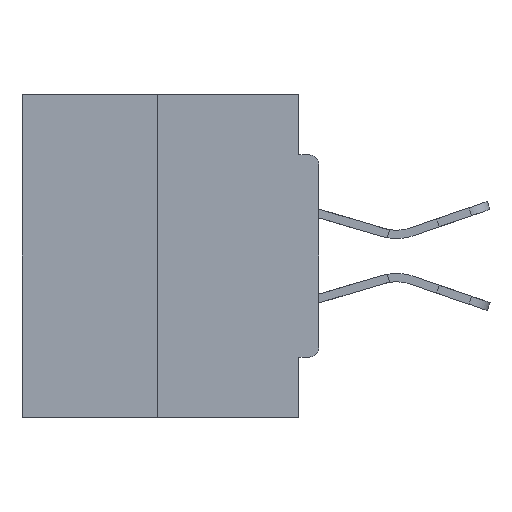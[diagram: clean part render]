
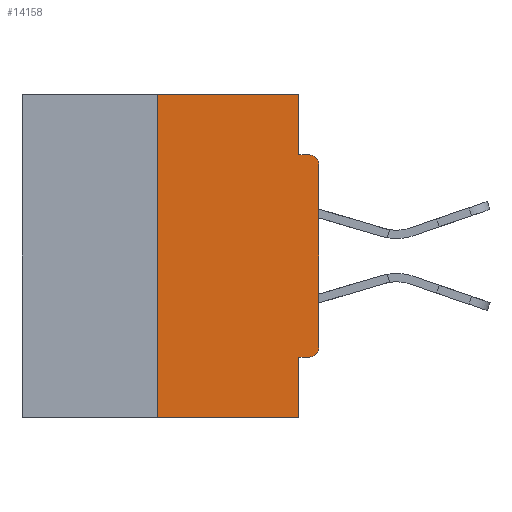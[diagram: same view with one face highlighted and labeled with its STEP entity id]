
A CAD part, left-side view. The second image highlights one B-rep face of the part: STEP entity #14158.
In plain terms, the highlighted planar face has unit normal (-1, 0, 0).
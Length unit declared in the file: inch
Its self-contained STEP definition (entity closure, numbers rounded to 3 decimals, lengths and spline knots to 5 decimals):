
#230 = ORIENTED_EDGE ( 'NONE', *, *, #789, .F. ) ;
#789 = EDGE_CURVE ( 'NONE', #2068, #12138, #25007, .T. ) ;
#1116 = VERTEX_POINT ( 'NONE', #14645 ) ;
#1739 = LINE ( 'NONE', #34316, #37080 ) ;
#1927 = CIRCLE ( 'NONE', #9295, 0.015 ) ;
#2068 = VERTEX_POINT ( 'NONE', #24907 ) ;
#2119 = DIRECTION ( 'NONE',  ( 0., 0., 1. ) ) ;
#2216 = EDGE_CURVE ( 'NONE', #1116, #17525, #6665, .T. ) ;
#2703 = EDGE_CURVE ( 'NONE', #25674, #12138, #1927, .T. ) ;
#2837 = CARTESIAN_POINT ( 'NONE',  ( 0., 0.25, 0. ) ) ;
#4883 = DIRECTION ( 'NONE',  ( -1., 0., 0. ) ) ;
#5009 = CARTESIAN_POINT ( 'NONE',  ( 0., 0., -0.4065 ) ) ;
#5109 = VECTOR ( 'NONE', #32019, 39.37008 ) ;
#5243 = ORIENTED_EDGE ( 'NONE', *, *, #34982, .T. ) ;
#5268 = DIRECTION ( 'NONE',  ( 0., 0., -1. ) ) ;
#5564 = ORIENTED_EDGE ( 'NONE', *, *, #30991, .F. ) ;
#6626 = ORIENTED_EDGE ( 'NONE', *, *, #29561, .T. ) ;
#6665 = LINE ( 'NONE', #30023, #23991 ) ;
#6961 = DIRECTION ( 'NONE',  ( 0., 0., -1. ) ) ;
#8534 = CARTESIAN_POINT ( 'NONE',  ( 0., 0.46, 0. ) ) ;
#9295 = AXIS2_PLACEMENT_3D ( 'NONE', #25380, #4883, #5268 ) ;
#9366 = DIRECTION ( 'NONE',  ( 0., 0., -1. ) ) ;
#9786 = EDGE_CURVE ( 'NONE', #11902, #2068, #20323, .T. ) ;
#11313 = ORIENTED_EDGE ( 'NONE', *, *, #35996, .T. ) ;
#11902 = VERTEX_POINT ( 'NONE', #14766 ) ;
#11984 = DIRECTION ( 'NONE',  ( 0., 0., -1. ) ) ;
#12138 = VERTEX_POINT ( 'NONE', #21803 ) ;
#12394 = CARTESIAN_POINT ( 'NONE',  ( 0., 0.031, -0.4065 ) ) ;
#12694 = ORIENTED_EDGE ( 'NONE', *, *, #2216, .F. ) ;
#12899 = PLANE ( 'NONE',  #28909 ) ;
#13634 = LINE ( 'NONE', #5009, #13907 ) ;
#13907 = VECTOR ( 'NONE', #25701, 39.37008 ) ;
#14158 = ADVANCED_FACE ( 'NONE', ( #21903 ), #12899, .F. ) ;
#14486 = DIRECTION ( 'NONE',  ( -1., 0., 0. ) ) ;
#14645 = CARTESIAN_POINT ( 'NONE',  ( 0., 0.25, -0.5 ) ) ;
#14766 = CARTESIAN_POINT ( 'NONE',  ( 0., 0.031, 0. ) ) ;
#15404 = CARTESIAN_POINT ( 'NONE',  ( 0., 0.46, 0. ) ) ;
#15468 = DIRECTION ( 'NONE',  ( 0., 0., 1. ) ) ;
#15965 = DIRECTION ( 'NONE',  ( 1., 0., 0. ) ) ;
#16001 = CARTESIAN_POINT ( 'NONE',  ( 0., 0., -0.0935 ) ) ;
#16078 = VECTOR ( 'NONE', #9366, 39.37008 ) ;
#16320 = VECTOR ( 'NONE', #20216, 39.37008 ) ;
#17525 = VERTEX_POINT ( 'NONE', #2837 ) ;
#17814 = LINE ( 'NONE', #29307, #16078 ) ;
#18212 = EDGE_CURVE ( 'NONE', #17525, #11902, #22536, .T. ) ;
#19085 = LINE ( 'NONE', #30772, #30173 ) ;
#20216 = DIRECTION ( 'NONE',  ( 0., -1., 0. ) ) ;
#20323 = LINE ( 'NONE', #26452, #5109 ) ;
#21071 = ORIENTED_EDGE ( 'NONE', *, *, #2703, .T. ) ;
#21586 = VERTEX_POINT ( 'NONE', #29163 ) ;
#21641 = CIRCLE ( 'NONE', #33888, 0.015 ) ;
#21744 = ORIENTED_EDGE ( 'NONE', *, *, #9786, .F. ) ;
#21803 = CARTESIAN_POINT ( 'NONE',  ( 0., 0.015, -0.0935 ) ) ;
#21903 = FACE_OUTER_BOUND ( 'NONE', #28185, .T. ) ;
#22145 = DIRECTION ( 'NONE',  ( 0., -1., 0. ) ) ;
#22536 = LINE ( 'NONE', #8534, #16320 ) ;
#23528 = VERTEX_POINT ( 'NONE', #29455 ) ;
#23991 = VECTOR ( 'NONE', #15468, 39.37008 ) ;
#24358 = ORIENTED_EDGE ( 'NONE', *, *, #34144, .F. ) ;
#24907 = CARTESIAN_POINT ( 'NONE',  ( 0., 0.031, -0.0935 ) ) ;
#25007 = LINE ( 'NONE', #16001, #30652 ) ;
#25380 = CARTESIAN_POINT ( 'NONE',  ( 0., 0.015, -0.1085 ) ) ;
#25674 = VERTEX_POINT ( 'NONE', #26966 ) ;
#25701 = DIRECTION ( 'NONE',  ( 0., 1., 0. ) ) ;
#26452 = CARTESIAN_POINT ( 'NONE',  ( 0., 0.031, 0. ) ) ;
#26966 = CARTESIAN_POINT ( 'NONE',  ( 0., 0., -0.1085 ) ) ;
#28185 = EDGE_LOOP ( 'NONE', ( #31526, #12694, #11313, #24358, #5564, #5243, #6626, #21071, #230, #21744 ) ) ;
#28909 = AXIS2_PLACEMENT_3D ( 'NONE', #15404, #15965, #6961 ) ;
#29163 = CARTESIAN_POINT ( 'NONE',  ( 0., 0.031, -0.5 ) ) ;
#29307 = CARTESIAN_POINT ( 'NONE',  ( 0., 0.031, -0.5 ) ) ;
#29455 = CARTESIAN_POINT ( 'NONE',  ( 0., 0., -0.3915 ) ) ;
#29561 = EDGE_CURVE ( 'NONE', #23528, #25674, #1739, .T. ) ;
#29848 = VERTEX_POINT ( 'NONE', #12394 ) ;
#30023 = CARTESIAN_POINT ( 'NONE',  ( 0., 0.25, 0. ) ) ;
#30173 = VECTOR ( 'NONE', #22145, 39.37008 ) ;
#30561 = DIRECTION ( 'NONE',  ( 0., -1., 0. ) ) ;
#30652 = VECTOR ( 'NONE', #30561, 39.37008 ) ;
#30772 = CARTESIAN_POINT ( 'NONE',  ( 0., 0.46, -0.5 ) ) ;
#30991 = EDGE_CURVE ( 'NONE', #33268, #29848, #13634, .T. ) ;
#31526 = ORIENTED_EDGE ( 'NONE', *, *, #18212, .F. ) ;
#32019 = DIRECTION ( 'NONE',  ( 0., 0., -1. ) ) ;
#32296 = CARTESIAN_POINT ( 'NONE',  ( 0., 0.015, -0.3915 ) ) ;
#33268 = VERTEX_POINT ( 'NONE', #34649 ) ;
#33888 = AXIS2_PLACEMENT_3D ( 'NONE', #32296, #14486, #11984 ) ;
#34144 = EDGE_CURVE ( 'NONE', #29848, #21586, #17814, .T. ) ;
#34316 = CARTESIAN_POINT ( 'NONE',  ( 0., 0., 0. ) ) ;
#34649 = CARTESIAN_POINT ( 'NONE',  ( 0., 0.015, -0.4065 ) ) ;
#34982 = EDGE_CURVE ( 'NONE', #33268, #23528, #21641, .T. ) ;
#35996 = EDGE_CURVE ( 'NONE', #1116, #21586, #19085, .T. ) ;
#37080 = VECTOR ( 'NONE', #2119, 39.37008 ) ;
